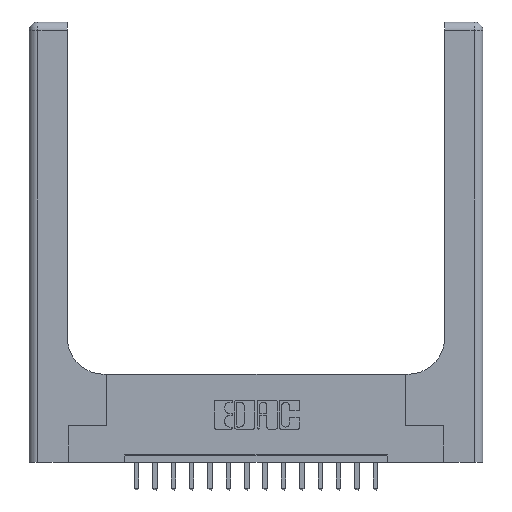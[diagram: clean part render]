
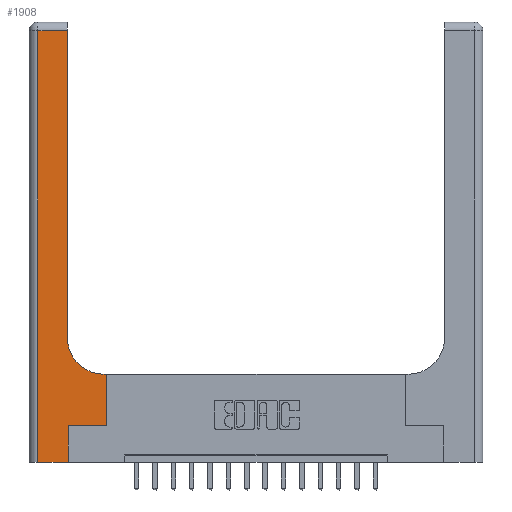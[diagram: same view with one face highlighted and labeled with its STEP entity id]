
A CAD part, top view. The second image highlights one B-rep face of the part: STEP entity #1908.
In plain terms, the highlighted planar face has unit normal (0, 0, 1).
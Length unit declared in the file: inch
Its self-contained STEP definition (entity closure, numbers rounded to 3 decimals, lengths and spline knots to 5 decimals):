
#68 = DIRECTION ( 'NONE',  ( 0., 1., 0. ) ) ;
#141 = CARTESIAN_POINT ( 'NONE',  ( 0., 3., 0.37 ) ) ;
#776 = LINE ( 'NONE', #6420, #15097 ) ;
#781 = CARTESIAN_POINT ( 'NONE',  ( 0.26, 2.94, 0.37 ) ) ;
#1219 = EDGE_CURVE ( 'NONE', #6061, #10811, #12584, .T. ) ;
#1254 = EDGE_CURVE ( 'NONE', #7378, #7407, #776, .T. ) ;
#1361 = DIRECTION ( 'NONE',  ( -1., 0., 0. ) ) ;
#1451 = LINE ( 'NONE', #5438, #10187 ) ;
#1537 = DIRECTION ( 'NONE',  ( -1., 0., 0. ) ) ;
#1908 = ADVANCED_FACE ( 'NONE', ( #7156 ), #12743, .F. ) ;
#1988 = ORIENTED_EDGE ( 'NONE', *, *, #15786, .T. ) ;
#2140 = EDGE_CURVE ( 'NONE', #10811, #14527, #9873, .T. ) ;
#2415 = CIRCLE ( 'NONE', #5643, 0.25 ) ;
#2538 = CARTESIAN_POINT ( 'NONE',  ( 0.51, 0.6, 0.37 ) ) ;
#2574 = DIRECTION ( 'NONE',  ( 1., 0., 0. ) ) ;
#2645 = VERTEX_POINT ( 'NONE', #9102 ) ;
#3025 = DIRECTION ( 'NONE',  ( 0., 0., -1. ) ) ;
#3245 = VERTEX_POINT ( 'NONE', #2538 ) ;
#3478 = CARTESIAN_POINT ( 'NONE',  ( 0.06, 2.94, 0.37 ) ) ;
#3591 = LINE ( 'NONE', #14581, #4230 ) ;
#4217 = CARTESIAN_POINT ( 'NONE',  ( 0.06, 0., 0.37 ) ) ;
#4230 = VECTOR ( 'NONE', #17717, 39.37008 ) ;
#4523 = DIRECTION ( 'NONE',  ( 1., 0., 0. ) ) ;
#5015 = ORIENTED_EDGE ( 'NONE', *, *, #5999, .T. ) ;
#5438 = CARTESIAN_POINT ( 'NONE',  ( 0.26, 0.6, 0.37 ) ) ;
#5476 = ORIENTED_EDGE ( 'NONE', *, *, #1219, .T. ) ;
#5480 = VECTOR ( 'NONE', #8260, 39.37008 ) ;
#5643 = AXIS2_PLACEMENT_3D ( 'NONE', #14133, #10027, #4523 ) ;
#5999 = EDGE_CURVE ( 'NONE', #13887, #2645, #14825, .T. ) ;
#6061 = VERTEX_POINT ( 'NONE', #3478 ) ;
#6284 = EDGE_LOOP ( 'NONE', ( #12322, #17590, #5476, #10898, #16927, #5015, #1988, #12744, #11261 ) ) ;
#6420 = CARTESIAN_POINT ( 'NONE',  ( 0.26, 3., 0.37 ) ) ;
#6790 = VERTEX_POINT ( 'NONE', #15011 ) ;
#6811 = DIRECTION ( 'NONE',  ( -1., 0., 0. ) ) ;
#7156 = FACE_OUTER_BOUND ( 'NONE', #6284, .T. ) ;
#7378 = VERTEX_POINT ( 'NONE', #12892 ) ;
#7407 = VERTEX_POINT ( 'NONE', #781 ) ;
#8260 = DIRECTION ( 'NONE',  ( 0., -1., 0. ) ) ;
#8554 = VECTOR ( 'NONE', #1537, 39.37008 ) ;
#9046 = EDGE_CURVE ( 'NONE', #14527, #13887, #18199, .T. ) ;
#9102 = CARTESIAN_POINT ( 'NONE',  ( 0.528, 0.25, 0.37 ) ) ;
#9292 = VECTOR ( 'NONE', #68, 39.37008 ) ;
#9686 = EDGE_CURVE ( 'NONE', #7407, #6061, #16949, .T. ) ;
#9776 = VECTOR ( 'NONE', #10832, 39.37008 ) ;
#9873 = LINE ( 'NONE', #14078, #10457 ) ;
#10027 = DIRECTION ( 'NONE',  ( 0., 0., -1. ) ) ;
#10187 = VECTOR ( 'NONE', #6811, 39.37008 ) ;
#10447 = CARTESIAN_POINT ( 'NONE',  ( 0.265, 0.25, 0.37 ) ) ;
#10457 = VECTOR ( 'NONE', #2574, 39.37008 ) ;
#10557 = EDGE_CURVE ( 'NONE', #3245, #7378, #2415, .T. ) ;
#10811 = VERTEX_POINT ( 'NONE', #4217 ) ;
#10832 = DIRECTION ( 'NONE',  ( 1., 0., 0. ) ) ;
#10898 = ORIENTED_EDGE ( 'NONE', *, *, #2140, .T. ) ;
#11138 = CARTESIAN_POINT ( 'NONE',  ( 0.265, 0.25, 0.37 ) ) ;
#11261 = ORIENTED_EDGE ( 'NONE', *, *, #10557, .T. ) ;
#12021 = EDGE_CURVE ( 'NONE', #6790, #3245, #1451, .T. ) ;
#12322 = ORIENTED_EDGE ( 'NONE', *, *, #1254, .T. ) ;
#12324 = CARTESIAN_POINT ( 'NONE',  ( 0.06, 3., 0.37 ) ) ;
#12584 = LINE ( 'NONE', #12324, #5480 ) ;
#12743 = PLANE ( 'NONE',  #12763 ) ;
#12744 = ORIENTED_EDGE ( 'NONE', *, *, #12021, .T. ) ;
#12763 = AXIS2_PLACEMENT_3D ( 'NONE', #141, #3025, #1361 ) ;
#12892 = CARTESIAN_POINT ( 'NONE',  ( 0.26, 0.85, 0.37 ) ) ;
#13887 = VERTEX_POINT ( 'NONE', #11138 ) ;
#14046 = CARTESIAN_POINT ( 'NONE',  ( 0.265, 0., 0.37 ) ) ;
#14078 = CARTESIAN_POINT ( 'NONE',  ( 0., 0., 0.37 ) ) ;
#14133 = CARTESIAN_POINT ( 'NONE',  ( 0.51, 0.85, 0.37 ) ) ;
#14527 = VERTEX_POINT ( 'NONE', #15259 ) ;
#14581 = CARTESIAN_POINT ( 'NONE',  ( 0.528, 0.25, 0.37 ) ) ;
#14825 = LINE ( 'NONE', #10447, #9776 ) ;
#15011 = CARTESIAN_POINT ( 'NONE',  ( 0.528, 0.6, 0.37 ) ) ;
#15097 = VECTOR ( 'NONE', #17222, 39.37008 ) ;
#15259 = CARTESIAN_POINT ( 'NONE',  ( 0.265, 0., 0.37 ) ) ;
#15485 = CARTESIAN_POINT ( 'NONE',  ( 0., 2.94, 0.37 ) ) ;
#15786 = EDGE_CURVE ( 'NONE', #2645, #6790, #3591, .T. ) ;
#16927 = ORIENTED_EDGE ( 'NONE', *, *, #9046, .T. ) ;
#16949 = LINE ( 'NONE', #15485, #8554 ) ;
#17222 = DIRECTION ( 'NONE',  ( 0., 1., 0. ) ) ;
#17590 = ORIENTED_EDGE ( 'NONE', *, *, #9686, .T. ) ;
#17717 = DIRECTION ( 'NONE',  ( 0., 1., 0. ) ) ;
#18199 = LINE ( 'NONE', #14046, #9292 ) ;
